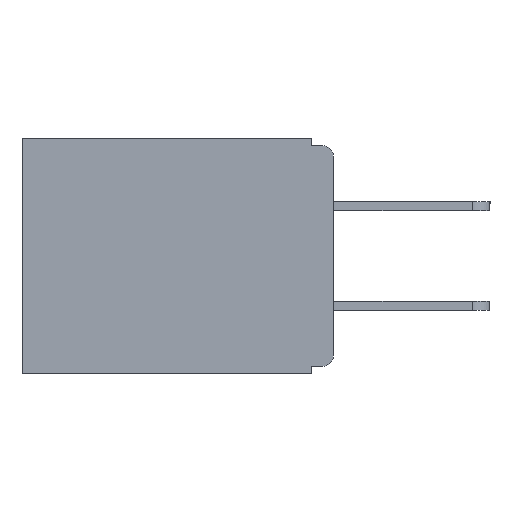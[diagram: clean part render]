
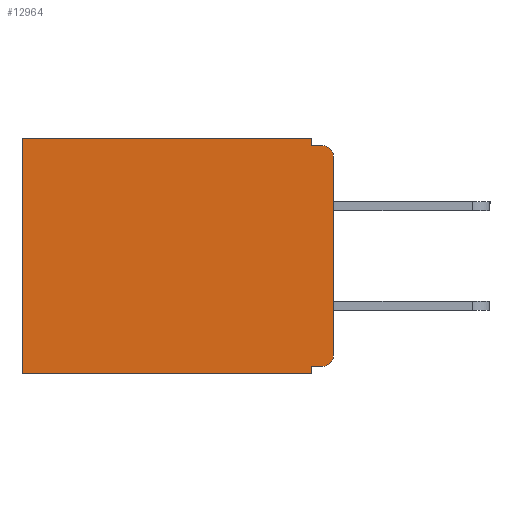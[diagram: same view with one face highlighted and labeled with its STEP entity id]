
A CAD part, left-side view. The second image highlights one B-rep face of the part: STEP entity #12964.
In plain terms, the highlighted planar face has unit normal (-1, 0, 0).
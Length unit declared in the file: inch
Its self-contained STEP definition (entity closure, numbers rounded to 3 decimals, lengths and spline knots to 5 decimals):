
#371 = LINE ( 'NONE', #25201, #15904 ) ;
#592 = ORIENTED_EDGE ( 'NONE', *, *, #5625, .F. ) ;
#642 = VERTEX_POINT ( 'NONE', #699 ) ;
#699 = CARTESIAN_POINT ( 'NONE',  ( 0.3, 0.015, -0.01 ) ) ;
#1153 = EDGE_CURVE ( 'NONE', #17207, #642, #25162, .T. ) ;
#1356 = ORIENTED_EDGE ( 'NONE', *, *, #23070, .T. ) ;
#1678 = DIRECTION ( 'NONE',  ( 1., 0., 0. ) ) ;
#1993 = VERTEX_POINT ( 'NONE', #21129 ) ;
#2010 = CIRCLE ( 'NONE', #10268, 0.015 ) ;
#2506 = CARTESIAN_POINT ( 'NONE',  ( 0.3, 0.437, -0.33 ) ) ;
#2542 = VERTEX_POINT ( 'NONE', #13528 ) ;
#2701 = CARTESIAN_POINT ( 'NONE',  ( 0.3, 0., -0.01 ) ) ;
#3554 = CARTESIAN_POINT ( 'NONE',  ( 0.3, 0.031, -0.33 ) ) ;
#3560 = VECTOR ( 'NONE', #25477, 39.37008 ) ;
#4021 = ORIENTED_EDGE ( 'NONE', *, *, #11912, .T. ) ;
#4251 = CARTESIAN_POINT ( 'NONE',  ( 0.3, 0., -0.32 ) ) ;
#4516 = EDGE_CURVE ( 'NONE', #6005, #14699, #19936, .T. ) ;
#4694 = DIRECTION ( 'NONE',  ( -1., 0., 0. ) ) ;
#4730 = EDGE_CURVE ( 'NONE', #20631, #7749, #10355, .T. ) ;
#5276 = VECTOR ( 'NONE', #10751, 39.37008 ) ;
#5389 = DIRECTION ( 'NONE',  ( 0., 0., -1. ) ) ;
#5583 = CARTESIAN_POINT ( 'NONE',  ( 0.3, 0., -0.33 ) ) ;
#5625 = EDGE_CURVE ( 'NONE', #7749, #2542, #371, .T. ) ;
#5925 = LINE ( 'NONE', #2701, #5276 ) ;
#6005 = VERTEX_POINT ( 'NONE', #15756 ) ;
#6157 = CARTESIAN_POINT ( 'NONE',  ( 0.3, 0.437, 0. ) ) ;
#6491 = ORIENTED_EDGE ( 'NONE', *, *, #6826, .F. ) ;
#6826 = EDGE_CURVE ( 'NONE', #1993, #20631, #12153, .T. ) ;
#7210 = DIRECTION ( 'NONE',  ( 0., 1., 0. ) ) ;
#7500 = DIRECTION ( 'NONE',  ( 0., 0., -1. ) ) ;
#7749 = VERTEX_POINT ( 'NONE', #3554 ) ;
#7871 = CARTESIAN_POINT ( 'NONE',  ( 0.3, 0., -0.33 ) ) ;
#8374 = ORIENTED_EDGE ( 'NONE', *, *, #4730, .F. ) ;
#9456 = VECTOR ( 'NONE', #7210, 39.37008 ) ;
#10268 = AXIS2_PLACEMENT_3D ( 'NONE', #16571, #4694, #18575 ) ;
#10355 = LINE ( 'NONE', #22060, #15029 ) ;
#10751 = DIRECTION ( 'NONE',  ( 0., -1., 0. ) ) ;
#11912 = EDGE_CURVE ( 'NONE', #14699, #2542, #25525, .T. ) ;
#11922 = ORIENTED_EDGE ( 'NONE', *, *, #17392, .F. ) ;
#12143 = CARTESIAN_POINT ( 'NONE',  ( 0.3, 0., -0.025 ) ) ;
#12153 = LINE ( 'NONE', #4251, #21380 ) ;
#12686 = VECTOR ( 'NONE', #7500, 39.37008 ) ;
#12964 = ADVANCED_FACE ( 'NONE', ( #24283 ), #25409, .F. ) ;
#13178 = ORIENTED_EDGE ( 'NONE', *, *, #1153, .T. ) ;
#13465 = DIRECTION ( 'NONE',  ( 0., 0., -1. ) ) ;
#13528 = CARTESIAN_POINT ( 'NONE',  ( 0.3, 0.437, -0.33 ) ) ;
#13613 = EDGE_LOOP ( 'NONE', ( #24137, #13178, #11922, #21175, #19941, #4021, #592, #8374, #6491, #1356 ) ) ;
#13664 = CARTESIAN_POINT ( 'NONE',  ( 0.3, 0.031, -0.32 ) ) ;
#14024 = CARTESIAN_POINT ( 'NONE',  ( 0.3, 0.015, -0.025 ) ) ;
#14199 = LINE ( 'NONE', #23565, #3560 ) ;
#14555 = DIRECTION ( 'NONE',  ( 0., 0., -1. ) ) ;
#14699 = VERTEX_POINT ( 'NONE', #6157 ) ;
#15029 = VECTOR ( 'NONE', #5389, 39.37008 ) ;
#15756 = CARTESIAN_POINT ( 'NONE',  ( 0.3, 0.031, 0. ) ) ;
#15787 = DIRECTION ( 'NONE',  ( 0., 0., -1. ) ) ;
#15904 = VECTOR ( 'NONE', #25173, 39.37008 ) ;
#16542 = AXIS2_PLACEMENT_3D ( 'NONE', #14024, #22994, #13465 ) ;
#16571 = CARTESIAN_POINT ( 'NONE',  ( 0.3, 0.015, -0.305 ) ) ;
#16959 = CARTESIAN_POINT ( 'NONE',  ( 0.3, 0., 0. ) ) ;
#17207 = VERTEX_POINT ( 'NONE', #12143 ) ;
#17392 = EDGE_CURVE ( 'NONE', #22072, #642, #5925, .T. ) ;
#18575 = DIRECTION ( 'NONE',  ( 0., 0., -1. ) ) ;
#19332 = EDGE_CURVE ( 'NONE', #6005, #22072, #14199, .T. ) ;
#19876 = VERTEX_POINT ( 'NONE', #21413 ) ;
#19936 = LINE ( 'NONE', #16959, #9456 ) ;
#19941 = ORIENTED_EDGE ( 'NONE', *, *, #4516, .T. ) ;
#20631 = VERTEX_POINT ( 'NONE', #13664 ) ;
#20851 = CARTESIAN_POINT ( 'NONE',  ( 0.3, 0.031, -0.01 ) ) ;
#21106 = VECTOR ( 'NONE', #14555, 39.37008 ) ;
#21129 = CARTESIAN_POINT ( 'NONE',  ( 0.3, 0.015, -0.32 ) ) ;
#21175 = ORIENTED_EDGE ( 'NONE', *, *, #19332, .F. ) ;
#21380 = VECTOR ( 'NONE', #23857, 39.37008 ) ;
#21413 = CARTESIAN_POINT ( 'NONE',  ( 0.3, 0., -0.305 ) ) ;
#22060 = CARTESIAN_POINT ( 'NONE',  ( 0.3, 0.031, -0.33 ) ) ;
#22072 = VERTEX_POINT ( 'NONE', #20851 ) ;
#22140 = AXIS2_PLACEMENT_3D ( 'NONE', #7871, #1678, #15787 ) ;
#22994 = DIRECTION ( 'NONE',  ( -1., 0., 0. ) ) ;
#23070 = EDGE_CURVE ( 'NONE', #1993, #19876, #2010, .T. ) ;
#23565 = CARTESIAN_POINT ( 'NONE',  ( 0.3, 0.031, 0. ) ) ;
#23636 = LINE ( 'NONE', #5583, #12686 ) ;
#23857 = DIRECTION ( 'NONE',  ( 0., 1., 0. ) ) ;
#24137 = ORIENTED_EDGE ( 'NONE', *, *, #25108, .F. ) ;
#24283 = FACE_OUTER_BOUND ( 'NONE', #13613, .T. ) ;
#25108 = EDGE_CURVE ( 'NONE', #17207, #19876, #23636, .T. ) ;
#25162 = CIRCLE ( 'NONE', #16542, 0.015 ) ;
#25173 = DIRECTION ( 'NONE',  ( 0., 1., 0. ) ) ;
#25201 = CARTESIAN_POINT ( 'NONE',  ( 0.3, 0., -0.33 ) ) ;
#25409 = PLANE ( 'NONE',  #22140 ) ;
#25477 = DIRECTION ( 'NONE',  ( 0., 0., -1. ) ) ;
#25525 = LINE ( 'NONE', #2506, #21106 ) ;
